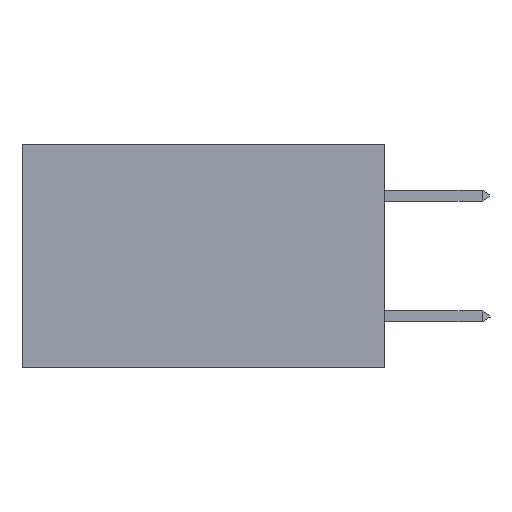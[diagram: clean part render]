
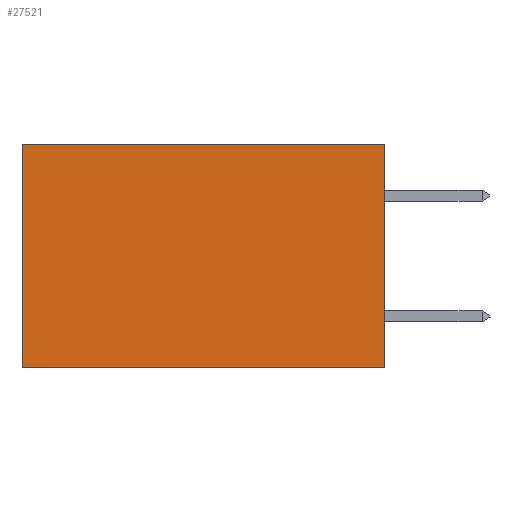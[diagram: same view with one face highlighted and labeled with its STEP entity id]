
A CAD part, left-side view. The second image highlights one B-rep face of the part: STEP entity #27521.
In plain terms, the highlighted planar face has unit normal (-1, 0, 0).
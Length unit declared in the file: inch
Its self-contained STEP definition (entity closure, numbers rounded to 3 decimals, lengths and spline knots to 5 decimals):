
#633 = CARTESIAN_POINT ( 'NONE',  ( 0.2875, 0., -0.37 ) ) ;
#1340 = ORIENTED_EDGE ( 'NONE', *, *, #22067, .F. ) ;
#2011 = EDGE_CURVE ( 'NONE', #6494, #18695, #23034, .T. ) ;
#4310 = CARTESIAN_POINT ( 'NONE',  ( 0.2875, 0.6, -0.37 ) ) ;
#5168 = LINE ( 'NONE', #24257, #28187 ) ;
#6494 = VERTEX_POINT ( 'NONE', #11233 ) ;
#6504 = EDGE_LOOP ( 'NONE', ( #27540, #12307, #1340, #14484 ) ) ;
#6837 = DIRECTION ( 'NONE',  ( 0., 0., -1. ) ) ;
#8266 = FACE_OUTER_BOUND ( 'NONE', #6504, .T. ) ;
#9287 = CARTESIAN_POINT ( 'NONE',  ( 0.2875, 0., 0. ) ) ;
#9604 = VECTOR ( 'NONE', #17811, 39.37008 ) ;
#10089 = DIRECTION ( 'NONE',  ( 0., 0., -1. ) ) ;
#11106 = VECTOR ( 'NONE', #23039, 39.37008 ) ;
#11233 = CARTESIAN_POINT ( 'NONE',  ( 0.2875, 0., -0.37 ) ) ;
#12227 = PLANE ( 'NONE',  #18661 ) ;
#12307 = ORIENTED_EDGE ( 'NONE', *, *, #2011, .F. ) ;
#14484 = ORIENTED_EDGE ( 'NONE', *, *, #28363, .T. ) ;
#14936 = CARTESIAN_POINT ( 'NONE',  ( 0.2875, 0., 0. ) ) ;
#16822 = CARTESIAN_POINT ( 'NONE',  ( 0.2875, 0., 0. ) ) ;
#17272 = LINE ( 'NONE', #14936, #9604 ) ;
#17811 = DIRECTION ( 'NONE',  ( 0., 1., 0. ) ) ;
#18661 = AXIS2_PLACEMENT_3D ( 'NONE', #16822, #25918, #10089 ) ;
#18695 = VERTEX_POINT ( 'NONE', #4310 ) ;
#18921 = CARTESIAN_POINT ( 'NONE',  ( 0.2875, 0.6, 0. ) ) ;
#19733 = DIRECTION ( 'NONE',  ( 0., 0., -1. ) ) ;
#19846 = EDGE_CURVE ( 'NONE', #20378, #18695, #5168, .T. ) ;
#20378 = VERTEX_POINT ( 'NONE', #18921 ) ;
#22067 = EDGE_CURVE ( 'NONE', #26883, #6494, #25840, .T. ) ;
#23034 = LINE ( 'NONE', #633, #11106 ) ;
#23039 = DIRECTION ( 'NONE',  ( 0., 1., 0. ) ) ;
#24257 = CARTESIAN_POINT ( 'NONE',  ( 0.2875, 0.6, 0. ) ) ;
#25840 = LINE ( 'NONE', #9287, #28631 ) ;
#25918 = DIRECTION ( 'NONE',  ( 1., 0., 0. ) ) ;
#26883 = VERTEX_POINT ( 'NONE', #27993 ) ;
#27521 = ADVANCED_FACE ( 'NONE', ( #8266 ), #12227, .F. ) ;
#27540 = ORIENTED_EDGE ( 'NONE', *, *, #19846, .T. ) ;
#27993 = CARTESIAN_POINT ( 'NONE',  ( 0.2875, 0., 0. ) ) ;
#28187 = VECTOR ( 'NONE', #19733, 39.37008 ) ;
#28363 = EDGE_CURVE ( 'NONE', #26883, #20378, #17272, .T. ) ;
#28631 = VECTOR ( 'NONE', #6837, 39.37008 ) ;
